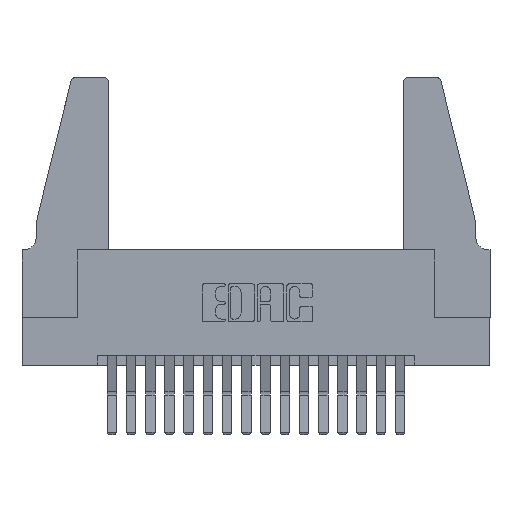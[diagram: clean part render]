
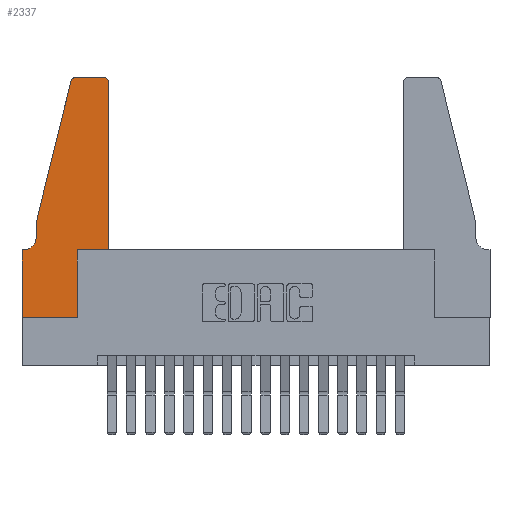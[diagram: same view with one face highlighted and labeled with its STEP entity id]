
A CAD part, top view. The second image highlights one B-rep face of the part: STEP entity #2337.
In plain terms, the highlighted planar face has unit normal (0, 0, 1).
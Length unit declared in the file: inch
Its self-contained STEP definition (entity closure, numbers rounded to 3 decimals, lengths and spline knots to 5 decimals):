
#18 = EDGE_CURVE ( 'NONE', #13722, #57, #8288, .T. ) ;
#53 = VECTOR ( 'NONE', #1219, 39.37008 ) ;
#57 = VERTEX_POINT ( 'NONE', #382 ) ;
#307 = LINE ( 'NONE', #5253, #15420 ) ;
#382 = CARTESIAN_POINT ( 'NONE',  ( 0.4205, 1.25, 0.37 ) ) ;
#397 = DIRECTION ( 'NONE',  ( -1., 0., 0. ) ) ;
#802 = AXIS2_PLACEMENT_3D ( 'NONE', #15931, #4568, #16119 ) ;
#812 = CARTESIAN_POINT ( 'NONE',  ( 0.2865, 0., 0.37 ) ) ;
#833 = CARTESIAN_POINT ( 'NONE',  ( 0.284, 1.22, 0.37 ) ) ;
#1219 = DIRECTION ( 'NONE',  ( 0., 1., 0. ) ) ;
#1251 = EDGE_CURVE ( 'NONE', #7067, #4055, #12310, .T. ) ;
#1298 = VECTOR ( 'NONE', #13379, 39.37008 ) ;
#1576 = EDGE_CURVE ( 'NONE', #15516, #3781, #10475, .T. ) ;
#1690 = DIRECTION ( 'NONE',  ( 0., 0., -1. ) ) ;
#1991 = DIRECTION ( 'NONE',  ( 1., 0., 0. ) ) ;
#2337 = ADVANCED_FACE ( 'NONE', ( #8273 ), #11910, .T. ) ;
#2420 = ORIENTED_EDGE ( 'NONE', *, *, #18, .T. ) ;
#2561 = CARTESIAN_POINT ( 'NONE',  ( 0.0755, 0.5, 0.37 ) ) ;
#2695 = VERTEX_POINT ( 'NONE', #16154 ) ;
#3243 = DIRECTION ( 'NONE',  ( 0., -1., 0. ) ) ;
#3552 = ORIENTED_EDGE ( 'NONE', *, *, #14622, .T. ) ;
#3561 = CARTESIAN_POINT ( 'NONE',  ( 0.0055, 0.35, 0.37 ) ) ;
#3570 = VERTEX_POINT ( 'NONE', #12005 ) ;
#3717 = DIRECTION ( 'NONE',  ( -1., 0., 0. ) ) ;
#3781 = VERTEX_POINT ( 'NONE', #812 ) ;
#3994 = CARTESIAN_POINT ( 'NONE',  ( 0.4505, 1.22, 0.37 ) ) ;
#4055 = VERTEX_POINT ( 'NONE', #3561 ) ;
#4568 = DIRECTION ( 'NONE',  ( 0., 0., 1. ) ) ;
#4731 = LINE ( 'NONE', #8656, #53 ) ;
#4916 = CARTESIAN_POINT ( 'NONE',  ( 0.4505, 0.35, 0.37 ) ) ;
#5209 = EDGE_CURVE ( 'NONE', #57, #6335, #6819, .T. ) ;
#5253 = CARTESIAN_POINT ( 'NONE',  ( 0.0755, 0.35, 0.37 ) ) ;
#5263 = CARTESIAN_POINT ( 'NONE',  ( 0.284, 1.25, 0.37 ) ) ;
#5282 = CARTESIAN_POINT ( 'NONE',  ( 0.4505, 0.35, 0.37 ) ) ;
#5424 = VECTOR ( 'NONE', #10184, 39.37008 ) ;
#6022 = CARTESIAN_POINT ( 'NONE',  ( 0.2865, 0.35, 0.37 ) ) ;
#6208 = CARTESIAN_POINT ( 'NONE',  ( 0., 0.35, 0.37 ) ) ;
#6335 = VERTEX_POINT ( 'NONE', #5263 ) ;
#6415 = VERTEX_POINT ( 'NONE', #6748 ) ;
#6605 = VECTOR ( 'NONE', #3717, 39.37008 ) ;
#6736 = ORIENTED_EDGE ( 'NONE', *, *, #17511, .T. ) ;
#6748 = CARTESIAN_POINT ( 'NONE',  ( 0.25487, 1.22718, 0.37 ) ) ;
#6819 = LINE ( 'NONE', #10745, #6605 ) ;
#6837 = EDGE_CURVE ( 'NONE', #7594, #2695, #16744, .T. ) ;
#7067 = VERTEX_POINT ( 'NONE', #16561 ) ;
#7112 = DIRECTION ( 'NONE',  ( 1., 0., 0. ) ) ;
#7484 = DIRECTION ( 'NONE',  ( 1., 0., 0. ) ) ;
#7492 = LINE ( 'NONE', #4916, #1298 ) ;
#7594 = VERTEX_POINT ( 'NONE', #6022 ) ;
#7600 = VECTOR ( 'NONE', #3243, 39.37008 ) ;
#7901 = ORIENTED_EDGE ( 'NONE', *, *, #5209, .T. ) ;
#8008 = CIRCLE ( 'NONE', #12009, 0.03 ) ;
#8273 = FACE_OUTER_BOUND ( 'NONE', #12850, .T. ) ;
#8288 = CIRCLE ( 'NONE', #802, 0.03 ) ;
#8497 = ORIENTED_EDGE ( 'NONE', *, *, #1576, .T. ) ;
#8656 = CARTESIAN_POINT ( 'NONE',  ( 0.2865, 0.35, 0.37 ) ) ;
#8757 = CARTESIAN_POINT ( 'NONE',  ( 0., 0., 0.37 ) ) ;
#8778 = VECTOR ( 'NONE', #13624, 39.37008 ) ;
#8896 = CARTESIAN_POINT ( 'NONE',  ( 0.0055, 0.42, 0.37 ) ) ;
#8963 = ORIENTED_EDGE ( 'NONE', *, *, #16013, .T. ) ;
#9719 = EDGE_CURVE ( 'NONE', #4055, #14471, #307, .T. ) ;
#10184 = DIRECTION ( 'NONE',  ( 1., 0., 0. ) ) ;
#10263 = EDGE_CURVE ( 'NONE', #6415, #3570, #14947, .T. ) ;
#10419 = DIRECTION ( 'NONE',  ( -1., 0., 0. ) ) ;
#10475 = LINE ( 'NONE', #8757, #5424 ) ;
#10745 = CARTESIAN_POINT ( 'NONE',  ( 0.2605, 1.25, 0.37 ) ) ;
#10855 = EDGE_CURVE ( 'NONE', #3781, #7594, #4731, .T. ) ;
#11618 = LINE ( 'NONE', #14477, #7600 ) ;
#11779 = ORIENTED_EDGE ( 'NONE', *, *, #6837, .T. ) ;
#11834 = CARTESIAN_POINT ( 'NONE',  ( 0., 0.35, 0.37 ) ) ;
#11910 = PLANE ( 'NONE',  #17672 ) ;
#11985 = ORIENTED_EDGE ( 'NONE', *, *, #9719, .T. ) ;
#12005 = CARTESIAN_POINT ( 'NONE',  ( 0.0755, 0.5, 0.37 ) ) ;
#12009 = AXIS2_PLACEMENT_3D ( 'NONE', #833, #17537, #1991 ) ;
#12082 = CARTESIAN_POINT ( 'NONE',  ( 0., 0., 0.37 ) ) ;
#12310 = CIRCLE ( 'NONE', #14688, 0.07 ) ;
#12455 = ORIENTED_EDGE ( 'NONE', *, *, #1251, .T. ) ;
#12582 = LINE ( 'NONE', #12082, #8778 ) ;
#12850 = EDGE_LOOP ( 'NONE', ( #7901, #6736, #15483, #8963, #12455, #11985, #3552, #8497, #18044, #11779, #15559, #2420 ) ) ;
#13015 = EDGE_CURVE ( 'NONE', #2695, #13722, #7492, .T. ) ;
#13379 = DIRECTION ( 'NONE',  ( 0., 1., 0. ) ) ;
#13391 = VECTOR ( 'NONE', #14048, 39.37008 ) ;
#13624 = DIRECTION ( 'NONE',  ( 0., -1., 0. ) ) ;
#13722 = VERTEX_POINT ( 'NONE', #3994 ) ;
#14048 = DIRECTION ( 'NONE',  ( -0.239, -0.971, 0. ) ) ;
#14471 = VERTEX_POINT ( 'NONE', #6208 ) ;
#14477 = CARTESIAN_POINT ( 'NONE',  ( 0.0755, 0.5, 0.37 ) ) ;
#14622 = EDGE_CURVE ( 'NONE', #14471, #15516, #12582, .T. ) ;
#14688 = AXIS2_PLACEMENT_3D ( 'NONE', #8896, #1690, #397 ) ;
#14947 = LINE ( 'NONE', #2561, #13391 ) ;
#15209 = VECTOR ( 'NONE', #7112, 39.37008 ) ;
#15420 = VECTOR ( 'NONE', #10419, 39.37008 ) ;
#15483 = ORIENTED_EDGE ( 'NONE', *, *, #10263, .T. ) ;
#15516 = VERTEX_POINT ( 'NONE', #16514 ) ;
#15559 = ORIENTED_EDGE ( 'NONE', *, *, #13015, .T. ) ;
#15931 = CARTESIAN_POINT ( 'NONE',  ( 0.4205, 1.22, 0.37 ) ) ;
#16013 = EDGE_CURVE ( 'NONE', #3570, #7067, #11618, .T. ) ;
#16119 = DIRECTION ( 'NONE',  ( 1., 0., 0. ) ) ;
#16154 = CARTESIAN_POINT ( 'NONE',  ( 0.4505, 0.35, 0.37 ) ) ;
#16514 = CARTESIAN_POINT ( 'NONE',  ( 0., 0., 0.37 ) ) ;
#16561 = CARTESIAN_POINT ( 'NONE',  ( 0.0755, 0.42, 0.37 ) ) ;
#16744 = LINE ( 'NONE', #5282, #15209 ) ;
#17436 = DIRECTION ( 'NONE',  ( 0., 0., 1. ) ) ;
#17511 = EDGE_CURVE ( 'NONE', #6335, #6415, #8008, .T. ) ;
#17537 = DIRECTION ( 'NONE',  ( 0., 0., 1. ) ) ;
#17672 = AXIS2_PLACEMENT_3D ( 'NONE', #11834, #17436, #7484 ) ;
#18044 = ORIENTED_EDGE ( 'NONE', *, *, #10855, .T. ) ;
